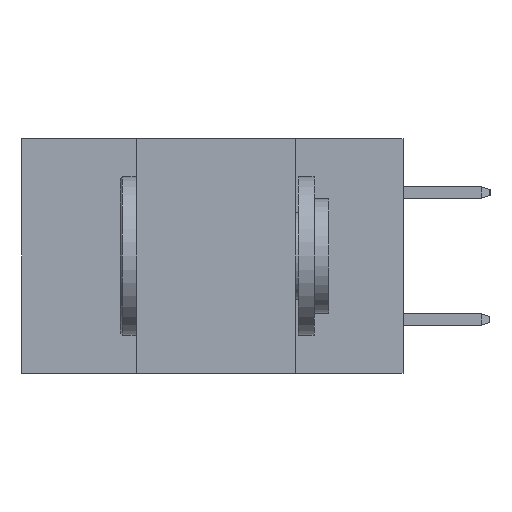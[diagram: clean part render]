
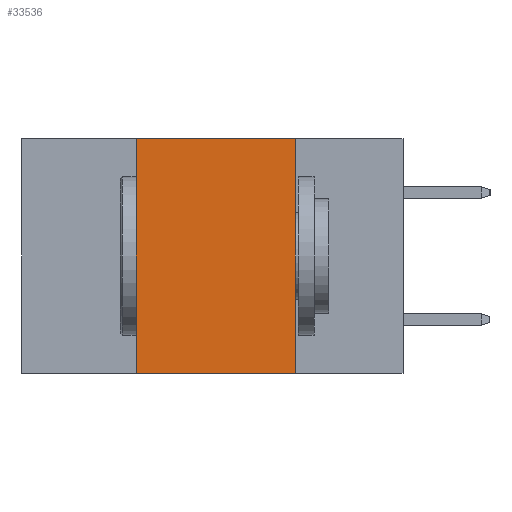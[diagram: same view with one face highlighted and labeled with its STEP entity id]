
A CAD part, left-side view. The second image highlights one B-rep face of the part: STEP entity #33536.
In plain terms, the highlighted planar face has unit normal (-1, 0, 0).
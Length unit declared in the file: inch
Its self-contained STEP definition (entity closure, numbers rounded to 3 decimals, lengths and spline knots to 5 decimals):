
#313 = CARTESIAN_POINT ( 'NONE',  ( 0., 0.6, 0. ) ) ;
#462 = CARTESIAN_POINT ( 'NONE',  ( 0., 0.42, -0.37 ) ) ;
#541 = CARTESIAN_POINT ( 'NONE',  ( 0., 0.17, 0. ) ) ;
#823 = ORIENTED_EDGE ( 'NONE', *, *, #46706, .T. ) ;
#2105 = DIRECTION ( 'NONE',  ( 0., -1., 0. ) ) ;
#2168 = VECTOR ( 'NONE', #40222, 39.37008 ) ;
#2950 = ORIENTED_EDGE ( 'NONE', *, *, #5349, .F. ) ;
#5349 = EDGE_CURVE ( 'NONE', #37015, #31374, #43128, .T. ) ;
#7187 = PLANE ( 'NONE',  #16464 ) ;
#7960 = EDGE_CURVE ( 'NONE', #8346, #41092, #44476, .T. ) ;
#8346 = VERTEX_POINT ( 'NONE', #541 ) ;
#9926 = CARTESIAN_POINT ( 'NONE',  ( 0., 0.6, 0. ) ) ;
#10613 = CARTESIAN_POINT ( 'NONE',  ( 0., 0.42, 0. ) ) ;
#10678 = ORIENTED_EDGE ( 'NONE', *, *, #7960, .F. ) ;
#11580 = CARTESIAN_POINT ( 'NONE',  ( 0., 0.17, -0.37 ) ) ;
#13245 = LINE ( 'NONE', #9926, #40333 ) ;
#14750 = DIRECTION ( 'NONE',  ( 0., 0., -1. ) ) ;
#15227 = FACE_OUTER_BOUND ( 'NONE', #32536, .T. ) ;
#15740 = CARTESIAN_POINT ( 'NONE',  ( 0., 0.17, 0. ) ) ;
#16464 = AXIS2_PLACEMENT_3D ( 'NONE', #313, #33264, #14750 ) ;
#16732 = CARTESIAN_POINT ( 'NONE',  ( 0., 0.6, -0.37 ) ) ;
#19757 = DIRECTION ( 'NONE',  ( 0., 0., -1. ) ) ;
#21829 = ORIENTED_EDGE ( 'NONE', *, *, #34335, .F. ) ;
#31374 = VERTEX_POINT ( 'NONE', #34977 ) ;
#32536 = EDGE_LOOP ( 'NONE', ( #10678, #21829, #2950, #823 ) ) ;
#33264 = DIRECTION ( 'NONE',  ( 1., 0., 0. ) ) ;
#33536 = ADVANCED_FACE ( 'NONE', ( #15227 ), #7187, .F. ) ;
#34090 = DIRECTION ( 'NONE',  ( 0., -1., 0. ) ) ;
#34319 = LINE ( 'NONE', #16732, #45362 ) ;
#34335 = EDGE_CURVE ( 'NONE', #31374, #8346, #13245, .T. ) ;
#34977 = CARTESIAN_POINT ( 'NONE',  ( 0., 0.42, 0. ) ) ;
#37015 = VERTEX_POINT ( 'NONE', #462 ) ;
#40222 = DIRECTION ( 'NONE',  ( 0., 0., 1. ) ) ;
#40333 = VECTOR ( 'NONE', #2105, 39.37008 ) ;
#41092 = VERTEX_POINT ( 'NONE', #11580 ) ;
#43128 = LINE ( 'NONE', #10613, #2168 ) ;
#43546 = VECTOR ( 'NONE', #19757, 39.37008 ) ;
#44476 = LINE ( 'NONE', #15740, #43546 ) ;
#45362 = VECTOR ( 'NONE', #34090, 39.37008 ) ;
#46706 = EDGE_CURVE ( 'NONE', #37015, #41092, #34319, .T. ) ;
